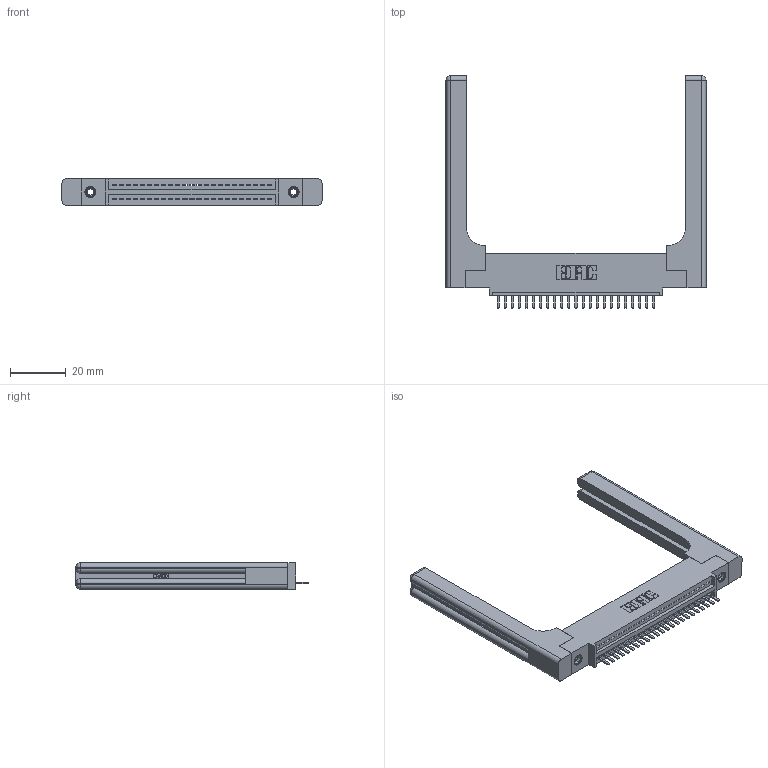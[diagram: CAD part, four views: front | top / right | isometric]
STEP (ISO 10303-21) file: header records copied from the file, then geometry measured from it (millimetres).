
FILE_DESCRIPTION (( 'STEP AP203' ), '1' );
FILE_NAME ('345-023-520-458.STEP', '2019-10-05T01:36:44', ( '' ), ( '' ), 'SwSTEP 2.0', 'SolidWorks 2016', '' );
FILE_SCHEMA (( 'CONFIG_CONTROL_DESIGN' ));
Length unit declared in the file: inch
Products named in the file (5): 345-220-058_345-220-058; 345-292-001_345-293-120; 345 Part_0.110 Offset - 0.156 Dia-TH; 345-023-520-458; 345-250-001_345-250-001-102
Assembly tree (28 placements, depth 2):
  345-023-520-458
    345 Part_0.110 Offset - 0.156 Dia-TH
    345-292-001_345-293-120  x23
    345-250-001_345-250-001-102  x2
    345-220-058_345-220-058  x2
Bounding box: 93.45 x 83.44 x 9.4 mm (x, y, z)
Volume: 17085.4 mm3; surface area: 16315.5 mm2
Topology: 28 solids, 28 shells, 1812 faces, 5251 edges, 3418 vertices
Faces by surface type: plane 1198, cylinder 554, bspline 36, cone 12, sphere 8, torus 4
Entity records: 25296 total; most frequent: CARTESIAN_POINT 5366, ORIENTED_EDGE 4108, DIRECTION 3648, EDGE_CURVE 2054, LINE 1734, VECTOR 1734, VERTEX_POINT 1358, AXIS2_PLACEMENT_3D 957
